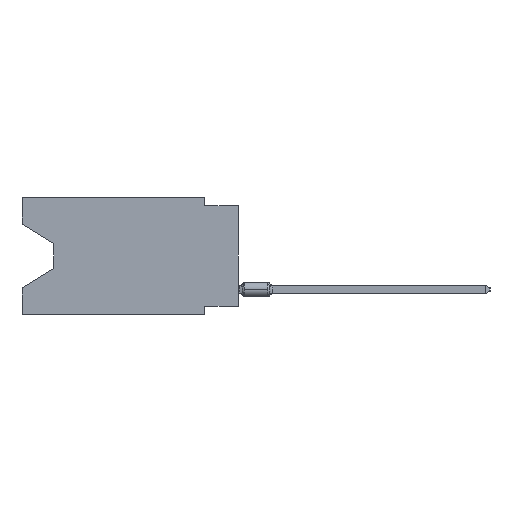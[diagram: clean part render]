
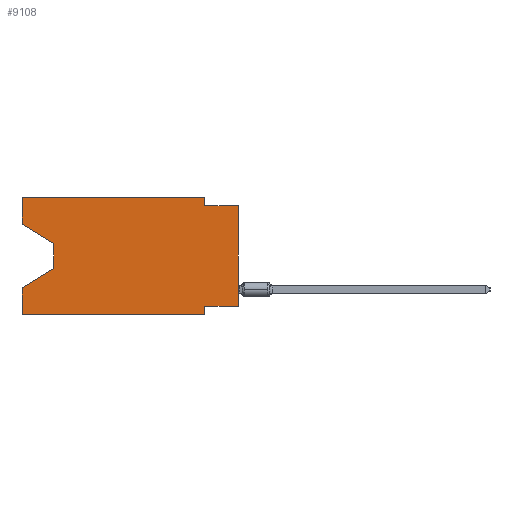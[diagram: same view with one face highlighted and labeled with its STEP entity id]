
A CAD part, left-side view. The second image highlights one B-rep face of the part: STEP entity #9108.
In plain terms, the highlighted planar face has unit normal (-1, 0, 0).
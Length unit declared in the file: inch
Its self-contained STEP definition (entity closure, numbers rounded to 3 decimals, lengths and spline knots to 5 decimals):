
#74 = LINE ( 'NONE', #29380, #37478 ) ;
#521 = CARTESIAN_POINT ( 'NONE',  ( 0., 0.55, -0.138 ) ) ;
#586 = ORIENTED_EDGE ( 'NONE', *, *, #28363, .T. ) ;
#642 = EDGE_CURVE ( 'NONE', #11603, #35844, #12616, .T. ) ;
#717 = VERTEX_POINT ( 'NONE', #36925 ) ;
#719 = CARTESIAN_POINT ( 'NONE',  ( 0., 0.645, 0. ) ) ;
#1537 = CARTESIAN_POINT ( 'NONE',  ( 0., 0.645, 0. ) ) ;
#1635 = EDGE_CURVE ( 'NONE', #25933, #27828, #15726, .T. ) ;
#2618 = EDGE_CURVE ( 'NONE', #22545, #18734, #43201, .T. ) ;
#3065 = DIRECTION ( 'NONE',  ( 0., 0., 1. ) ) ;
#3686 = DIRECTION ( 'NONE',  ( 0., 0., -1. ) ) ;
#4193 = LINE ( 'NONE', #18842, #28970 ) ;
#6429 = ORIENTED_EDGE ( 'NONE', *, *, #2618, .T. ) ;
#6610 = VECTOR ( 'NONE', #19633, 39.37008 ) ;
#6835 = VECTOR ( 'NONE', #45416, 39.37008 ) ;
#7084 = VECTOR ( 'NONE', #3065, 39.37008 ) ;
#7489 = FACE_OUTER_BOUND ( 'NONE', #46893, .T. ) ;
#8281 = DIRECTION ( 'NONE',  ( 0., -1., 0. ) ) ;
#8690 = VERTEX_POINT ( 'NONE', #26487 ) ;
#9108 = ADVANCED_FACE ( 'NONE', ( #7489 ), #25736, .F. ) ;
#10429 = CARTESIAN_POINT ( 'NONE',  ( 0., 0.1, -0.025 ) ) ;
#11091 = ORIENTED_EDGE ( 'NONE', *, *, #24801, .F. ) ;
#11113 = CARTESIAN_POINT ( 'NONE',  ( 0., 0.645, 0. ) ) ;
#11603 = VERTEX_POINT ( 'NONE', #27080 ) ;
#12616 = LINE ( 'NONE', #1537, #25400 ) ;
#12914 = ORIENTED_EDGE ( 'NONE', *, *, #39943, .T. ) ;
#13268 = VECTOR ( 'NONE', #41875, 39.37008 ) ;
#13971 = EDGE_CURVE ( 'NONE', #36439, #11603, #30748, .T. ) ;
#14702 = VECTOR ( 'NONE', #46813, 39.37008 ) ;
#14763 = LINE ( 'NONE', #521, #16825 ) ;
#14879 = EDGE_CURVE ( 'NONE', #717, #22545, #14763, .T. ) ;
#15113 = DIRECTION ( 'NONE',  ( 0., 0., 1. ) ) ;
#15726 = LINE ( 'NONE', #16191, #13268 ) ;
#16191 = CARTESIAN_POINT ( 'NONE',  ( 0., 0.1, -0.35 ) ) ;
#16825 = VECTOR ( 'NONE', #3686, 39.37008 ) ;
#16962 = CARTESIAN_POINT ( 'NONE',  ( 0., 0.645, -0.08025 ) ) ;
#17326 = CARTESIAN_POINT ( 'NONE',  ( 0., 0.1, 0. ) ) ;
#17494 = CARTESIAN_POINT ( 'NONE',  ( 0., 0.55, -0.212 ) ) ;
#17886 = EDGE_CURVE ( 'NONE', #8690, #25933, #19165, .T. ) ;
#18734 = VERTEX_POINT ( 'NONE', #44969 ) ;
#18842 = CARTESIAN_POINT ( 'NONE',  ( 0., 0., -0.025 ) ) ;
#19165 = LINE ( 'NONE', #41744, #6610 ) ;
#19240 = DIRECTION ( 'NONE',  ( 0., 0., -1. ) ) ;
#19633 = DIRECTION ( 'NONE',  ( 0., 1., 0. ) ) ;
#19695 = EDGE_CURVE ( 'NONE', #36439, #717, #74, .T. ) ;
#20028 = ORIENTED_EDGE ( 'NONE', *, *, #19695, .T. ) ;
#20360 = DIRECTION ( 'NONE',  ( 0., -1., 0. ) ) ;
#21191 = CARTESIAN_POINT ( 'NONE',  ( 0., 0.1, -0.35 ) ) ;
#22267 = DIRECTION ( 'NONE',  ( 0., -1., 0. ) ) ;
#22545 = VERTEX_POINT ( 'NONE', #25559 ) ;
#22791 = ORIENTED_EDGE ( 'NONE', *, *, #17886, .F. ) ;
#24772 = CARTESIAN_POINT ( 'NONE',  ( 0., 0.645, -0.35 ) ) ;
#24801 = EDGE_CURVE ( 'NONE', #35844, #46816, #25005, .T. ) ;
#25005 = LINE ( 'NONE', #17326, #26864 ) ;
#25400 = VECTOR ( 'NONE', #22267, 39.37008 ) ;
#25559 = CARTESIAN_POINT ( 'NONE',  ( 0., 0.55, -0.212 ) ) ;
#25736 = PLANE ( 'NONE',  #30272 ) ;
#25933 = VERTEX_POINT ( 'NONE', #38266 ) ;
#26487 = CARTESIAN_POINT ( 'NONE',  ( 0., 0., -0.325 ) ) ;
#26864 = VECTOR ( 'NONE', #36062, 39.37008 ) ;
#27080 = CARTESIAN_POINT ( 'NONE',  ( 0., 0.645, 0. ) ) ;
#27828 = VERTEX_POINT ( 'NONE', #21191 ) ;
#28015 = CARTESIAN_POINT ( 'NONE',  ( 0., 0.645, -0.35 ) ) ;
#28363 = EDGE_CURVE ( 'NONE', #8690, #40069, #37909, .T. ) ;
#28519 = CARTESIAN_POINT ( 'NONE',  ( 0., 0.645, 0. ) ) ;
#28610 = EDGE_CURVE ( 'NONE', #37206, #18734, #47267, .T. ) ;
#28970 = VECTOR ( 'NONE', #8281, 39.37008 ) ;
#29119 = CARTESIAN_POINT ( 'NONE',  ( 0., 0.1, 0. ) ) ;
#29380 = CARTESIAN_POINT ( 'NONE',  ( 0., 0.645, -0.08025 ) ) ;
#30272 = AXIS2_PLACEMENT_3D ( 'NONE', #11113, #44711, #19240 ) ;
#30748 = LINE ( 'NONE', #719, #6835 ) ;
#32465 = EDGE_CURVE ( 'NONE', #46816, #40069, #4193, .T. ) ;
#33700 = DIRECTION ( 'NONE',  ( 0., -0.855, -0.519 ) ) ;
#34152 = ORIENTED_EDGE ( 'NONE', *, *, #1635, .F. ) ;
#34654 = VECTOR ( 'NONE', #15113, 39.37008 ) ;
#35844 = VERTEX_POINT ( 'NONE', #29119 ) ;
#36062 = DIRECTION ( 'NONE',  ( 0., 0., -1. ) ) ;
#36439 = VERTEX_POINT ( 'NONE', #16962 ) ;
#36850 = ORIENTED_EDGE ( 'NONE', *, *, #642, .F. ) ;
#36925 = CARTESIAN_POINT ( 'NONE',  ( 0., 0.55, -0.138 ) ) ;
#37206 = VERTEX_POINT ( 'NONE', #24772 ) ;
#37478 = VECTOR ( 'NONE', #33700, 39.37008 ) ;
#37631 = ORIENTED_EDGE ( 'NONE', *, *, #32465, .F. ) ;
#37909 = LINE ( 'NONE', #40812, #34654 ) ;
#38266 = CARTESIAN_POINT ( 'NONE',  ( 0., 0.1, -0.325 ) ) ;
#39706 = ORIENTED_EDGE ( 'NONE', *, *, #14879, .T. ) ;
#39811 = CARTESIAN_POINT ( 'NONE',  ( 0., 0., -0.025 ) ) ;
#39943 = EDGE_CURVE ( 'NONE', #37206, #27828, #46320, .T. ) ;
#40069 = VERTEX_POINT ( 'NONE', #39811 ) ;
#40812 = CARTESIAN_POINT ( 'NONE',  ( 0., 0., 0. ) ) ;
#41744 = CARTESIAN_POINT ( 'NONE',  ( 0., 0., -0.325 ) ) ;
#41875 = DIRECTION ( 'NONE',  ( 0., 0., -1. ) ) ;
#42740 = VECTOR ( 'NONE', #20360, 39.37008 ) ;
#43201 = LINE ( 'NONE', #17494, #14702 ) ;
#43573 = ORIENTED_EDGE ( 'NONE', *, *, #28610, .F. ) ;
#44711 = DIRECTION ( 'NONE',  ( 1., 0., 0. ) ) ;
#44969 = CARTESIAN_POINT ( 'NONE',  ( 0., 0.645, -0.26975 ) ) ;
#45416 = DIRECTION ( 'NONE',  ( 0., 0., 1. ) ) ;
#45500 = ORIENTED_EDGE ( 'NONE', *, *, #13971, .F. ) ;
#46320 = LINE ( 'NONE', #28015, #42740 ) ;
#46813 = DIRECTION ( 'NONE',  ( 0., 0.855, -0.519 ) ) ;
#46816 = VERTEX_POINT ( 'NONE', #10429 ) ;
#46893 = EDGE_LOOP ( 'NONE', ( #20028, #39706, #6429, #43573, #12914, #34152, #22791, #586, #37631, #11091, #36850, #45500 ) ) ;
#47267 = LINE ( 'NONE', #28519, #7084 ) ;
